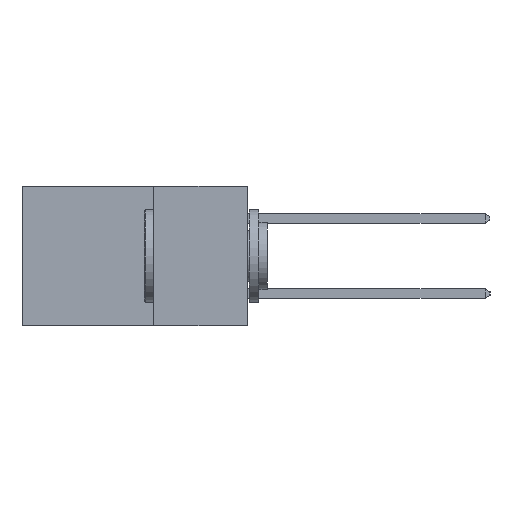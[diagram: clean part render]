
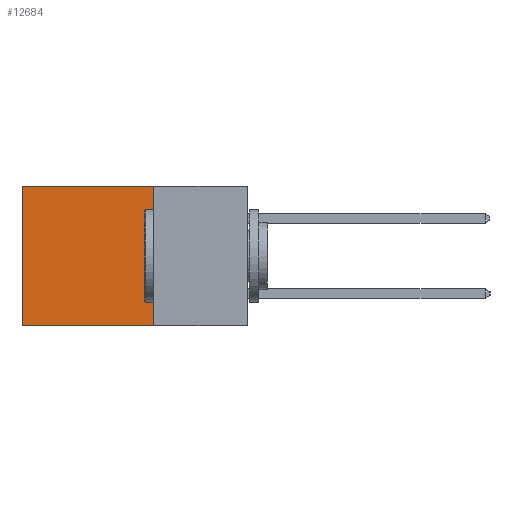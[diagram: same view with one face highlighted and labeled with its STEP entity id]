
A CAD part, left-side view. The second image highlights one B-rep face of the part: STEP entity #12684.
In plain terms, the highlighted planar face has unit normal (-1, 0, 0).
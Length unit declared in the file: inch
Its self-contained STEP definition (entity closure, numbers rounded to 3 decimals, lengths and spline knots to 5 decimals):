
#427 = VERTEX_POINT ( 'NONE', #15911 ) ;
#2503 = VECTOR ( 'NONE', #14447, 39.37008 ) ;
#3123 = CARTESIAN_POINT ( 'NONE',  ( 0.2615, 0.6, -0.37 ) ) ;
#3310 = ORIENTED_EDGE ( 'NONE', *, *, #12518, .T. ) ;
#3319 = FACE_OUTER_BOUND ( 'NONE', #14431, .T. ) ;
#4705 = EDGE_CURVE ( 'NONE', #9903, #10969, #21663, .T. ) ;
#4820 = CARTESIAN_POINT ( 'NONE',  ( 0.2615, 0.25, -0.37 ) ) ;
#6085 = AXIS2_PLACEMENT_3D ( 'NONE', #18328, #21816, #11378 ) ;
#7080 = VECTOR ( 'NONE', #22202, 39.37008 ) ;
#7357 = EDGE_CURVE ( 'NONE', #15559, #427, #14021, .T. ) ;
#8630 = ORIENTED_EDGE ( 'NONE', *, *, #21097, .F. ) ;
#9903 = VERTEX_POINT ( 'NONE', #21334 ) ;
#10969 = VERTEX_POINT ( 'NONE', #3123 ) ;
#11378 = DIRECTION ( 'NONE',  ( 0., 0., -1. ) ) ;
#12518 = EDGE_CURVE ( 'NONE', #15559, #9903, #21617, .T. ) ;
#12684 = ADVANCED_FACE ( 'NONE', ( #3319 ), #20092, .F. ) ;
#12909 = DIRECTION ( 'NONE',  ( 0., 0., -1. ) ) ;
#12935 = CARTESIAN_POINT ( 'NONE',  ( 0.2615, 0.6, -0.37 ) ) ;
#13735 = ORIENTED_EDGE ( 'NONE', *, *, #7357, .F. ) ;
#14021 = LINE ( 'NONE', #16940, #18090 ) ;
#14431 = EDGE_LOOP ( 'NONE', ( #17947, #8630, #13735, #3310 ) ) ;
#14447 = DIRECTION ( 'NONE',  ( 0., 1., 0. ) ) ;
#15559 = VERTEX_POINT ( 'NONE', #22521 ) ;
#15911 = CARTESIAN_POINT ( 'NONE',  ( 0.2615, 0.25, -0.37 ) ) ;
#16342 = LINE ( 'NONE', #4820, #7080 ) ;
#16916 = DIRECTION ( 'NONE',  ( 0., 0., -1. ) ) ;
#16940 = CARTESIAN_POINT ( 'NONE',  ( 0.2615, 0.25, -0.37 ) ) ;
#17947 = ORIENTED_EDGE ( 'NONE', *, *, #4705, .T. ) ;
#17961 = CARTESIAN_POINT ( 'NONE',  ( 0.2615, 0.25, 0. ) ) ;
#18090 = VECTOR ( 'NONE', #16916, 39.37008 ) ;
#18328 = CARTESIAN_POINT ( 'NONE',  ( 0.2615, 0.25, -0.37 ) ) ;
#20092 = PLANE ( 'NONE',  #6085 ) ;
#21097 = EDGE_CURVE ( 'NONE', #427, #10969, #16342, .T. ) ;
#21334 = CARTESIAN_POINT ( 'NONE',  ( 0.2615, 0.6, 0. ) ) ;
#21617 = LINE ( 'NONE', #17961, #2503 ) ;
#21663 = LINE ( 'NONE', #12935, #22194 ) ;
#21816 = DIRECTION ( 'NONE',  ( 1., 0., 0. ) ) ;
#22194 = VECTOR ( 'NONE', #12909, 39.37008 ) ;
#22202 = DIRECTION ( 'NONE',  ( 0., 1., 0. ) ) ;
#22521 = CARTESIAN_POINT ( 'NONE',  ( 0.2615, 0.25, 0. ) ) ;
